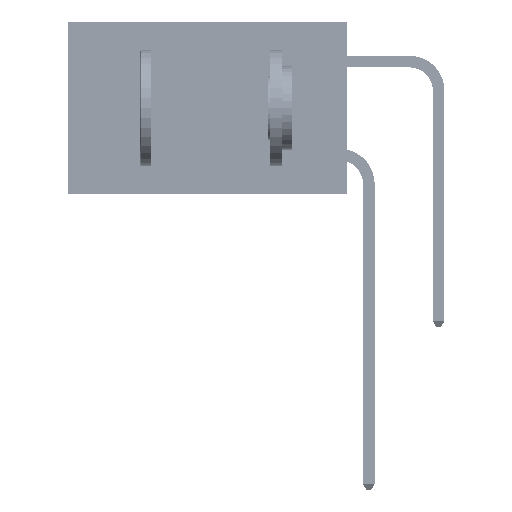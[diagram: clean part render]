
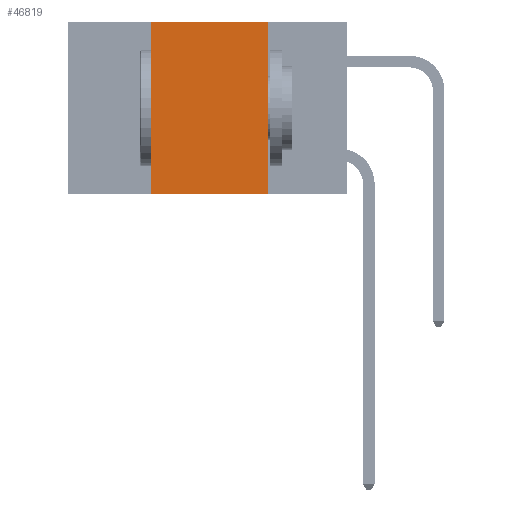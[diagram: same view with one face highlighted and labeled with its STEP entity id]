
A CAD part, left-side view. The second image highlights one B-rep face of the part: STEP entity #46819.
In plain terms, the highlighted planar face has unit normal (-1, 0, 0).
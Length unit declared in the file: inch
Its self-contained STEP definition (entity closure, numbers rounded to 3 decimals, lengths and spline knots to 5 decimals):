
#427 = DIRECTION ( 'NONE',  ( 1., 0., 0. ) ) ;
#10869 = EDGE_CURVE ( 'NONE', #34184, #33494, #31607, .T. ) ;
#13320 = CARTESIAN_POINT ( 'NONE',  ( 0., 0.17, 0. ) ) ;
#16259 = CARTESIAN_POINT ( 'NONE',  ( 0., 0.6, 0. ) ) ;
#16976 = CARTESIAN_POINT ( 'NONE',  ( 0., 0.6, -0.37 ) ) ;
#18021 = CARTESIAN_POINT ( 'NONE',  ( 0., 0.17, -0.37 ) ) ;
#18261 = DIRECTION ( 'NONE',  ( 0., -1., 0. ) ) ;
#18820 = VECTOR ( 'NONE', #20987, 39.37008 ) ;
#19216 = CARTESIAN_POINT ( 'NONE',  ( 0., 0.42, -0.37 ) ) ;
#20987 = DIRECTION ( 'NONE',  ( 0., 0., -1. ) ) ;
#22216 = ORIENTED_EDGE ( 'NONE', *, *, #37262, .T. ) ;
#25995 = CARTESIAN_POINT ( 'NONE',  ( 0., 0.17, 0. ) ) ;
#26723 = VERTEX_POINT ( 'NONE', #42250 ) ;
#27899 = EDGE_LOOP ( 'NONE', ( #45129, #35553, #31331, #22216 ) ) ;
#28021 = DIRECTION ( 'NONE',  ( 0., 0., -1. ) ) ;
#29230 = LINE ( 'NONE', #37606, #48333 ) ;
#29857 = EDGE_CURVE ( 'NONE', #26723, #34184, #29230, .T. ) ;
#30965 = VECTOR ( 'NONE', #32629, 39.37008 ) ;
#31331 = ORIENTED_EDGE ( 'NONE', *, *, #42997, .F. ) ;
#31590 = DIRECTION ( 'NONE',  ( 0., 0., 1. ) ) ;
#31607 = LINE ( 'NONE', #13320, #18820 ) ;
#32629 = DIRECTION ( 'NONE',  ( 0., -1., 0. ) ) ;
#33157 = VECTOR ( 'NONE', #31590, 39.37008 ) ;
#33494 = VERTEX_POINT ( 'NONE', #18021 ) ;
#34184 = VERTEX_POINT ( 'NONE', #25995 ) ;
#35553 = ORIENTED_EDGE ( 'NONE', *, *, #29857, .F. ) ;
#37262 = EDGE_CURVE ( 'NONE', #42307, #33494, #50048, .T. ) ;
#37606 = CARTESIAN_POINT ( 'NONE',  ( 0., 0.6, 0. ) ) ;
#39331 = CARTESIAN_POINT ( 'NONE',  ( 0., 0.42, 0. ) ) ;
#39473 = PLANE ( 'NONE',  #42884 ) ;
#42250 = CARTESIAN_POINT ( 'NONE',  ( 0., 0.42, 0. ) ) ;
#42307 = VERTEX_POINT ( 'NONE', #19216 ) ;
#42884 = AXIS2_PLACEMENT_3D ( 'NONE', #16259, #427, #28021 ) ;
#42997 = EDGE_CURVE ( 'NONE', #42307, #26723, #43280, .T. ) ;
#43280 = LINE ( 'NONE', #39331, #33157 ) ;
#45129 = ORIENTED_EDGE ( 'NONE', *, *, #10869, .F. ) ;
#46819 = ADVANCED_FACE ( 'NONE', ( #48161 ), #39473, .F. ) ;
#48161 = FACE_OUTER_BOUND ( 'NONE', #27899, .T. ) ;
#48333 = VECTOR ( 'NONE', #18261, 39.37008 ) ;
#50048 = LINE ( 'NONE', #16976, #30965 ) ;
